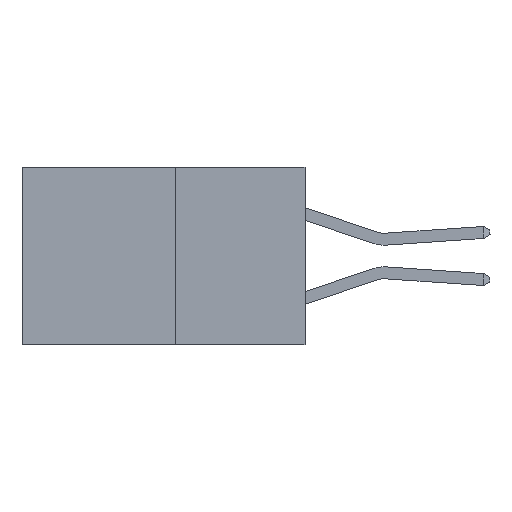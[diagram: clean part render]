
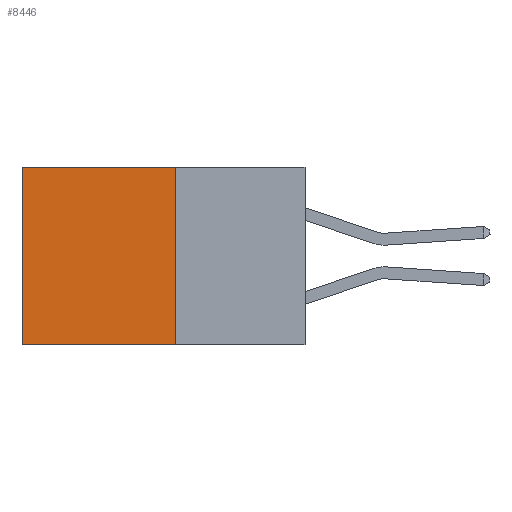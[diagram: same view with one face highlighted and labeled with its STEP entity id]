
A CAD part, left-side view. The second image highlights one B-rep face of the part: STEP entity #8446.
In plain terms, the highlighted planar face has unit normal (-1, 0, 0).
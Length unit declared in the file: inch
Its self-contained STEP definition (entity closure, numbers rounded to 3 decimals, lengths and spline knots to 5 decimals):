
#116 = CARTESIAN_POINT ( 'NONE',  ( 0.277, 0.27, -0.37 ) ) ;
#1021 = VECTOR ( 'NONE', #15831, 39.37008 ) ;
#2456 = VERTEX_POINT ( 'NONE', #11646 ) ;
#4011 = LINE ( 'NONE', #21451, #17338 ) ;
#4527 = CARTESIAN_POINT ( 'NONE',  ( 0.277, 0.27, -0.37 ) ) ;
#4778 = LINE ( 'NONE', #4801, #17037 ) ;
#4801 = CARTESIAN_POINT ( 'NONE',  ( 0.277, 0.27, -0.37 ) ) ;
#6302 = DIRECTION ( 'NONE',  ( 0., 0., -1. ) ) ;
#6536 = ORIENTED_EDGE ( 'NONE', *, *, #15484, .T. ) ;
#6850 = ORIENTED_EDGE ( 'NONE', *, *, #9141, .F. ) ;
#7138 = EDGE_LOOP ( 'NONE', ( #6536, #13422, #6850, #18914 ) ) ;
#7168 = CARTESIAN_POINT ( 'NONE',  ( 0.277, 0.27, -0.37 ) ) ;
#7301 = EDGE_CURVE ( 'NONE', #8351, #2456, #17676, .T. ) ;
#7412 = EDGE_CURVE ( 'NONE', #11840, #21607, #14965, .T. ) ;
#7863 = VECTOR ( 'NONE', #13790, 39.37008 ) ;
#8351 = VERTEX_POINT ( 'NONE', #11250 ) ;
#8446 = ADVANCED_FACE ( 'NONE', ( #17333 ), #11483, .F. ) ;
#9141 = EDGE_CURVE ( 'NONE', #8351, #11840, #4778, .T. ) ;
#9347 = DIRECTION ( 'NONE',  ( 0., 0., -1. ) ) ;
#11250 = CARTESIAN_POINT ( 'NONE',  ( 0.277, 0.27, 0. ) ) ;
#11483 = PLANE ( 'NONE',  #16708 ) ;
#11646 = CARTESIAN_POINT ( 'NONE',  ( 0.277, 0.59, 0. ) ) ;
#11840 = VERTEX_POINT ( 'NONE', #7168 ) ;
#13422 = ORIENTED_EDGE ( 'NONE', *, *, #7412, .F. ) ;
#13790 = DIRECTION ( 'NONE',  ( 0., 1., 0. ) ) ;
#14965 = LINE ( 'NONE', #116, #1021 ) ;
#15248 = DIRECTION ( 'NONE',  ( 0., 0., -1. ) ) ;
#15484 = EDGE_CURVE ( 'NONE', #2456, #21607, #4011, .T. ) ;
#15831 = DIRECTION ( 'NONE',  ( 0., 1., 0. ) ) ;
#16708 = AXIS2_PLACEMENT_3D ( 'NONE', #4527, #16713, #6302 ) ;
#16713 = DIRECTION ( 'NONE',  ( 1., 0., 0. ) ) ;
#17037 = VECTOR ( 'NONE', #15248, 39.37008 ) ;
#17333 = FACE_OUTER_BOUND ( 'NONE', #7138, .T. ) ;
#17338 = VECTOR ( 'NONE', #9347, 39.37008 ) ;
#17676 = LINE ( 'NONE', #22411, #7863 ) ;
#18896 = CARTESIAN_POINT ( 'NONE',  ( 0.277, 0.59, -0.37 ) ) ;
#18914 = ORIENTED_EDGE ( 'NONE', *, *, #7301, .T. ) ;
#21451 = CARTESIAN_POINT ( 'NONE',  ( 0.277, 0.59, -0.37 ) ) ;
#21607 = VERTEX_POINT ( 'NONE', #18896 ) ;
#22411 = CARTESIAN_POINT ( 'NONE',  ( 0.277, 0.27, 0. ) ) ;
